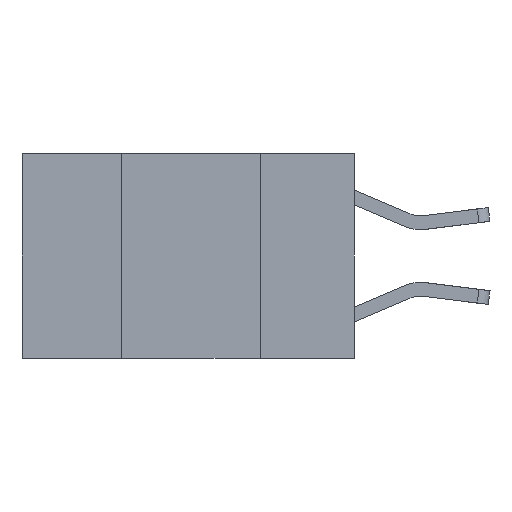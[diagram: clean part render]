
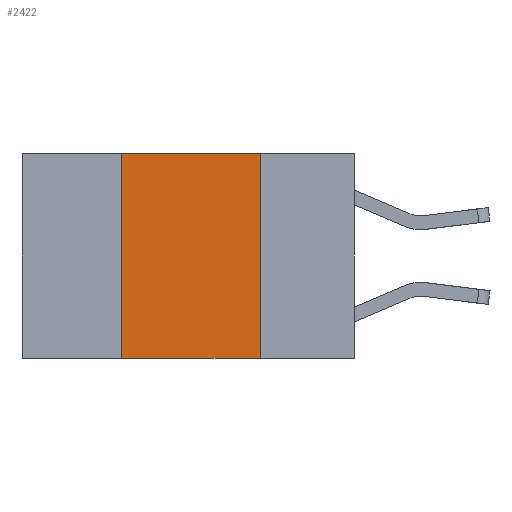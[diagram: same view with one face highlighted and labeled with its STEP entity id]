
A CAD part, left-side view. The second image highlights one B-rep face of the part: STEP entity #2422.
In plain terms, the highlighted planar face has unit normal (-1, 0, 0).
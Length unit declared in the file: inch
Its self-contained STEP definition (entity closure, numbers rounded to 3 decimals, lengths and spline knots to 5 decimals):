
#32 = ORIENTED_EDGE ( 'NONE', *, *, #4728, .F. ) ;
#657 = ORIENTED_EDGE ( 'NONE', *, *, #5817, .F. ) ;
#658 = LINE ( 'NONE', #10953, #5966 ) ;
#906 = CARTESIAN_POINT ( 'NONE',  ( 0., 0.6, 0. ) ) ;
#2015 = VECTOR ( 'NONE', #6573, 39.37008 ) ;
#2422 = ADVANCED_FACE ( 'NONE', ( #12142 ), #3908, .F. ) ;
#3386 = VECTOR ( 'NONE', #6339, 39.37008 ) ;
#3589 = CARTESIAN_POINT ( 'NONE',  ( 0., 0.17, 0. ) ) ;
#3769 = CARTESIAN_POINT ( 'NONE',  ( 0., 0.17, -0.37 ) ) ;
#3908 = PLANE ( 'NONE',  #12969 ) ;
#3921 = DIRECTION ( 'NONE',  ( 0., -1., 0. ) ) ;
#4355 = VERTEX_POINT ( 'NONE', #11076 ) ;
#4728 = EDGE_CURVE ( 'NONE', #7471, #6005, #7677, .T. ) ;
#5284 = VECTOR ( 'NONE', #7336, 39.37008 ) ;
#5817 = EDGE_CURVE ( 'NONE', #8340, #4355, #7999, .T. ) ;
#5911 = DIRECTION ( 'NONE',  ( 0., 0., -1. ) ) ;
#5964 = ORIENTED_EDGE ( 'NONE', *, *, #9071, .T. ) ;
#5966 = VECTOR ( 'NONE', #3921, 39.37008 ) ;
#6005 = VERTEX_POINT ( 'NONE', #3769 ) ;
#6339 = DIRECTION ( 'NONE',  ( 0., -1., 0. ) ) ;
#6382 = EDGE_CURVE ( 'NONE', #4355, #7471, #8765, .T. ) ;
#6573 = DIRECTION ( 'NONE',  ( 0., 0., -1. ) ) ;
#7336 = DIRECTION ( 'NONE',  ( 0., 0., 1. ) ) ;
#7471 = VERTEX_POINT ( 'NONE', #12995 ) ;
#7677 = LINE ( 'NONE', #3589, #2015 ) ;
#7999 = LINE ( 'NONE', #12352, #5284 ) ;
#8340 = VERTEX_POINT ( 'NONE', #10666 ) ;
#8765 = LINE ( 'NONE', #10405, #3386 ) ;
#9071 = EDGE_CURVE ( 'NONE', #8340, #6005, #658, .T. ) ;
#10405 = CARTESIAN_POINT ( 'NONE',  ( 0., 0.6, 0. ) ) ;
#10666 = CARTESIAN_POINT ( 'NONE',  ( 0., 0.42, -0.37 ) ) ;
#10707 = ORIENTED_EDGE ( 'NONE', *, *, #6382, .F. ) ;
#10953 = CARTESIAN_POINT ( 'NONE',  ( 0., 0.6, -0.37 ) ) ;
#11076 = CARTESIAN_POINT ( 'NONE',  ( 0., 0.42, 0. ) ) ;
#11971 = DIRECTION ( 'NONE',  ( 1., 0., 0. ) ) ;
#12142 = FACE_OUTER_BOUND ( 'NONE', #13001, .T. ) ;
#12352 = CARTESIAN_POINT ( 'NONE',  ( 0., 0.42, 0. ) ) ;
#12969 = AXIS2_PLACEMENT_3D ( 'NONE', #906, #11971, #5911 ) ;
#12995 = CARTESIAN_POINT ( 'NONE',  ( 0., 0.17, 0. ) ) ;
#13001 = EDGE_LOOP ( 'NONE', ( #32, #10707, #657, #5964 ) ) ;
